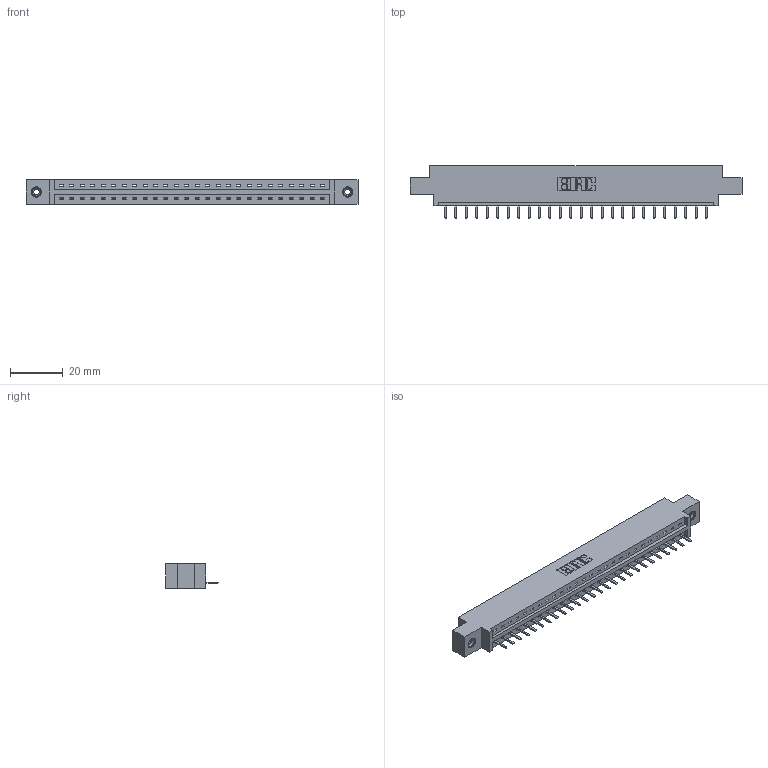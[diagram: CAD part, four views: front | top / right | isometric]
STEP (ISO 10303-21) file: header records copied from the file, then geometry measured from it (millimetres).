
FILE_DESCRIPTION (( 'STEP AP203' ), '1' );
FILE_NAME ('337-026-520-608.STEP', '2019-09-30T18:19:30', ( '' ), ( '' ), 'SwSTEP 2.0', 'SolidWorks 2016', '' );
FILE_SCHEMA (( 'CONFIG_CONTROL_DESIGN' ));
Length unit declared in the file: inch
Products named in the file (4): 345-250-001_345-250-003-102; 337-026-520-608; 345-292-001_345-293-120; 337 Part_0.170 Offset - 0.156 Dia-TI
Assembly tree (29 placements, depth 2):
  337-026-520-608
    337 Part_0.170 Offset - 0.156 Dia-TI
    345-292-001_345-293-120  x26
    345-250-001_345-250-003-102  x2
Bounding box: 126.03 x 20.02 x 9.4 mm (x, y, z)
Volume: 12700.2 mm3; surface area: 12891.9 mm2
Topology: 29 solids, 29 shells, 1894 faces, 5555 edges, 3626 vertices
Faces by surface type: plane 1354, cylinder 524, cone 12, torus 4
Entity records: 22828 total; most frequent: CARTESIAN_POINT 3967, ORIENTED_EDGE 3910, DIRECTION 3393, EDGE_CURVE 1955, VECTOR 1803, LINE 1803, VERTEX_POINT 1296, AXIS2_PLACEMENT_3D 795
